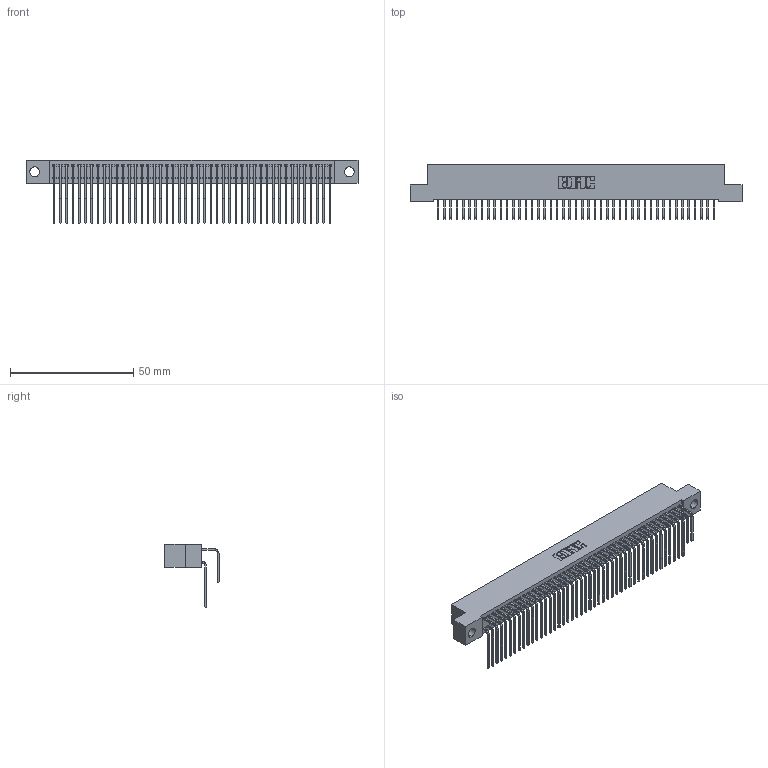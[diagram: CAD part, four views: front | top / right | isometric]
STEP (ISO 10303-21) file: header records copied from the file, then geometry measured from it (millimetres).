
FILE_DESCRIPTION (( 'STEP AP203' ), '1' );
FILE_NAME ('392-090-558-204.STEP', '2018-08-18T07:25:06', ( '' ), ( '' ), 'SwSTEP 2.0', 'SolidWorks 2016', '' );
FILE_SCHEMA (( 'CONFIG_CONTROL_DESIGN' ));
Length unit declared in the file: inch
Products named in the file (4): 345-292-001_558 559 Tail - 1; 345-292-001_558 Tail - 2; 392-090-558-204; 342 Part_.156 TH
Assembly tree (91 placements, depth 2):
  392-090-558-204
    342 Part_.156 TH
    345-292-001_558 559 Tail - 1  x45
    345-292-001_558 Tail - 2  x45
Bounding box: 134.62 x 21.91 x 25.78 mm (x, y, z)
Volume: 12541.9 mm3; surface area: 22661.9 mm2
Topology: 91 solids, 91 shells, 4970 faces, 14789 edges, 9738 vertices
Faces by surface type: plane 3486, cylinder 1484
Entity records: 30217 total; most frequent: CARTESIAN_POINT 5053, ORIENTED_EDGE 4938, DIRECTION 4293, EDGE_CURVE 2469, LINE 2301, VECTOR 2301, VERTEX_POINT 1642, AXIS2_PLACEMENT_3D 996
